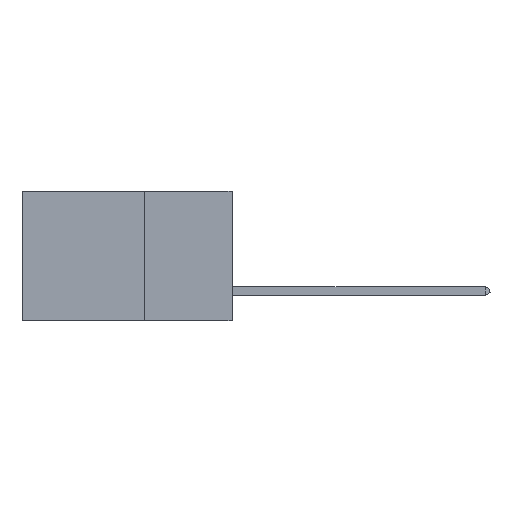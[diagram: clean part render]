
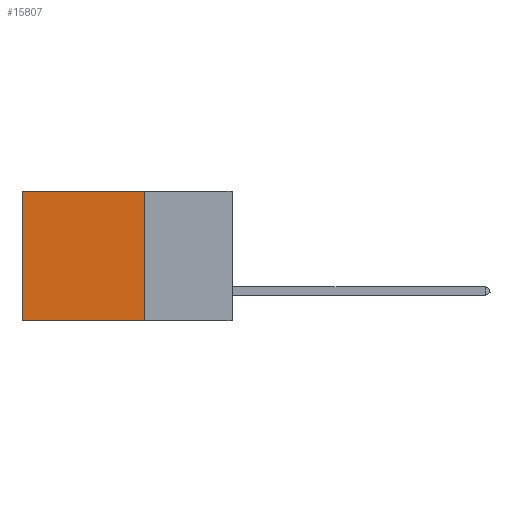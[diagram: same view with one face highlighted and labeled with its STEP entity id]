
A CAD part, left-side view. The second image highlights one B-rep face of the part: STEP entity #15807.
In plain terms, the highlighted planar face has unit normal (-1, 0, 0).
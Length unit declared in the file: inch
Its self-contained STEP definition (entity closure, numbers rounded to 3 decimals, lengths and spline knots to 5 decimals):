
#211 = EDGE_CURVE ( 'NONE', #9124, #10045, #25457, .T. ) ;
#3941 = AXIS2_PLACEMENT_3D ( 'NONE', #20977, #24568, #34505 ) ;
#5239 = VERTEX_POINT ( 'NONE', #19251 ) ;
#7629 = CARTESIAN_POINT ( 'NONE',  ( 0.2875, 0.6, 0. ) ) ;
#8716 = CARTESIAN_POINT ( 'NONE',  ( 0.2875, 0.25, 0. ) ) ;
#9077 = VECTOR ( 'NONE', #16385, 39.37008 ) ;
#9124 = VERTEX_POINT ( 'NONE', #8716 ) ;
#10045 = VERTEX_POINT ( 'NONE', #13475 ) ;
#11572 = PLANE ( 'NONE',  #3941 ) ;
#11961 = VECTOR ( 'NONE', #28246, 39.37008 ) ;
#12094 = ORIENTED_EDGE ( 'NONE', *, *, #16727, .F. ) ;
#13475 = CARTESIAN_POINT ( 'NONE',  ( 0.2875, 0.6, 0. ) ) ;
#13779 = CARTESIAN_POINT ( 'NONE',  ( 0.2875, 0.25, 0. ) ) ;
#14455 = EDGE_CURVE ( 'NONE', #10045, #36176, #29451, .T. ) ;
#15807 = ADVANCED_FACE ( 'NONE', ( #39256 ), #11572, .F. ) ;
#16385 = DIRECTION ( 'NONE',  ( 0., 1., 0. ) ) ;
#16667 = CARTESIAN_POINT ( 'NONE',  ( 0.2875, 0.25, -0.37 ) ) ;
#16727 = EDGE_CURVE ( 'NONE', #9124, #5239, #36070, .T. ) ;
#19251 = CARTESIAN_POINT ( 'NONE',  ( 0.2875, 0.25, -0.37 ) ) ;
#19505 = ORIENTED_EDGE ( 'NONE', *, *, #211, .T. ) ;
#19700 = EDGE_LOOP ( 'NONE', ( #39151, #23552, #12094, #19505 ) ) ;
#20977 = CARTESIAN_POINT ( 'NONE',  ( 0.2875, 0.25, 0. ) ) ;
#22519 = EDGE_CURVE ( 'NONE', #5239, #36176, #23682, .T. ) ;
#23552 = ORIENTED_EDGE ( 'NONE', *, *, #22519, .F. ) ;
#23682 = LINE ( 'NONE', #16667, #41764 ) ;
#23914 = DIRECTION ( 'NONE',  ( 0., 0., -1. ) ) ;
#24568 = DIRECTION ( 'NONE',  ( 1., 0., 0. ) ) ;
#25457 = LINE ( 'NONE', #13779, #9077 ) ;
#28246 = DIRECTION ( 'NONE',  ( 0., 0., -1. ) ) ;
#29451 = LINE ( 'NONE', #7629, #32015 ) ;
#32015 = VECTOR ( 'NONE', #23914, 39.37008 ) ;
#33162 = DIRECTION ( 'NONE',  ( 0., 1., 0. ) ) ;
#34505 = DIRECTION ( 'NONE',  ( 0., 0., -1. ) ) ;
#34665 = CARTESIAN_POINT ( 'NONE',  ( 0.2875, 0.6, -0.37 ) ) ;
#36070 = LINE ( 'NONE', #41799, #11961 ) ;
#36176 = VERTEX_POINT ( 'NONE', #34665 ) ;
#39151 = ORIENTED_EDGE ( 'NONE', *, *, #14455, .T. ) ;
#39256 = FACE_OUTER_BOUND ( 'NONE', #19700, .T. ) ;
#41764 = VECTOR ( 'NONE', #33162, 39.37008 ) ;
#41799 = CARTESIAN_POINT ( 'NONE',  ( 0.2875, 0.25, 0. ) ) ;
